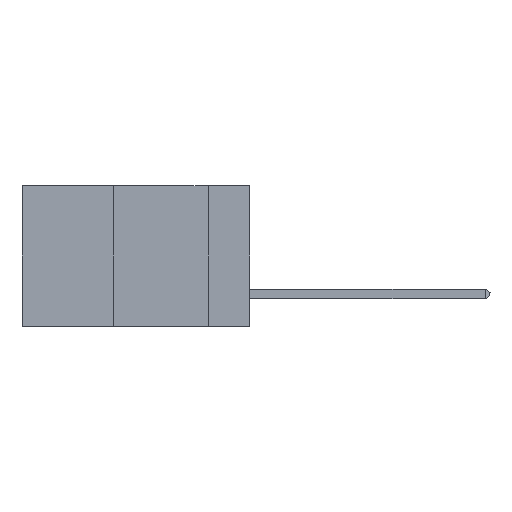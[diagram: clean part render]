
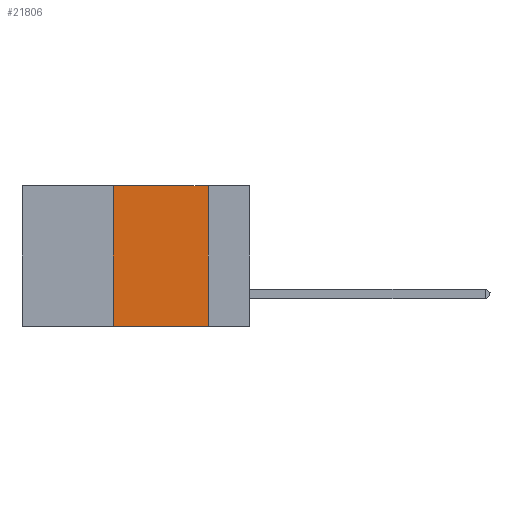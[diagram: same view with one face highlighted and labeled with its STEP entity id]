
A CAD part, left-side view. The second image highlights one B-rep face of the part: STEP entity #21806.
In plain terms, the highlighted planar face has unit normal (-1, 0, 0).
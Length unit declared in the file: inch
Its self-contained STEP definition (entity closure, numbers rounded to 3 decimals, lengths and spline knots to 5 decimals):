
#426 = VECTOR ( 'NONE', #38489, 39.37008 ) ;
#1471 = CARTESIAN_POINT ( 'NONE',  ( 0., 0.11, 0. ) ) ;
#2430 = VECTOR ( 'NONE', #30299, 39.37008 ) ;
#3831 = CARTESIAN_POINT ( 'NONE',  ( 0., 0.36, 0. ) ) ;
#4267 = VERTEX_POINT ( 'NONE', #15392 ) ;
#4804 = DIRECTION ( 'NONE',  ( 0., 0., -1. ) ) ;
#6840 = DIRECTION ( 'NONE',  ( 0., 0., -1. ) ) ;
#8223 = LINE ( 'NONE', #25753, #426 ) ;
#8521 = EDGE_CURVE ( 'NONE', #4267, #41260, #8223, .T. ) ;
#9888 = DIRECTION ( 'NONE',  ( 1., 0., 0. ) ) ;
#10034 = CARTESIAN_POINT ( 'NONE',  ( 0., 0.6, 0. ) ) ;
#10681 = EDGE_CURVE ( 'NONE', #42313, #39091, #29101, .T. ) ;
#11696 = CARTESIAN_POINT ( 'NONE',  ( 0., 0.6, 0. ) ) ;
#13018 = EDGE_CURVE ( 'NONE', #4267, #42313, #14394, .T. ) ;
#13089 = LINE ( 'NONE', #1471, #29630 ) ;
#14394 = LINE ( 'NONE', #3831, #2430 ) ;
#15392 = CARTESIAN_POINT ( 'NONE',  ( 0., 0.36, -0.37 ) ) ;
#16215 = ORIENTED_EDGE ( 'NONE', *, *, #13018, .F. ) ;
#18185 = DIRECTION ( 'NONE',  ( 0., -1., 0. ) ) ;
#20207 = FACE_OUTER_BOUND ( 'NONE', #35921, .T. ) ;
#21806 = ADVANCED_FACE ( 'NONE', ( #20207 ), #39828, .F. ) ;
#21887 = ORIENTED_EDGE ( 'NONE', *, *, #10681, .F. ) ;
#25060 = CARTESIAN_POINT ( 'NONE',  ( 0., 0.11, 0. ) ) ;
#25753 = CARTESIAN_POINT ( 'NONE',  ( 0., 0.6, -0.37 ) ) ;
#26000 = VECTOR ( 'NONE', #18185, 39.37008 ) ;
#26193 = EDGE_CURVE ( 'NONE', #39091, #41260, #13089, .T. ) ;
#29101 = LINE ( 'NONE', #11696, #26000 ) ;
#29630 = VECTOR ( 'NONE', #4804, 39.37008 ) ;
#29966 = CARTESIAN_POINT ( 'NONE',  ( 0., 0.11, -0.37 ) ) ;
#30299 = DIRECTION ( 'NONE',  ( 0., 0., 1. ) ) ;
#30473 = ORIENTED_EDGE ( 'NONE', *, *, #26193, .F. ) ;
#32467 = AXIS2_PLACEMENT_3D ( 'NONE', #10034, #9888, #6840 ) ;
#34786 = CARTESIAN_POINT ( 'NONE',  ( 0., 0.36, 0. ) ) ;
#35921 = EDGE_LOOP ( 'NONE', ( #30473, #21887, #16215, #36217 ) ) ;
#36217 = ORIENTED_EDGE ( 'NONE', *, *, #8521, .T. ) ;
#38489 = DIRECTION ( 'NONE',  ( 0., -1., 0. ) ) ;
#39091 = VERTEX_POINT ( 'NONE', #25060 ) ;
#39828 = PLANE ( 'NONE',  #32467 ) ;
#41260 = VERTEX_POINT ( 'NONE', #29966 ) ;
#42313 = VERTEX_POINT ( 'NONE', #34786 ) ;
